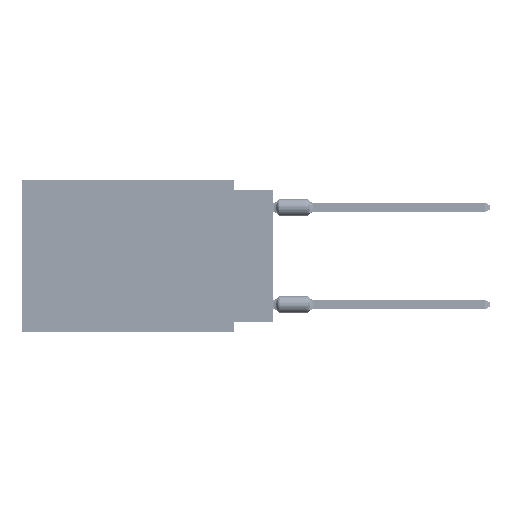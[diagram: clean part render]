
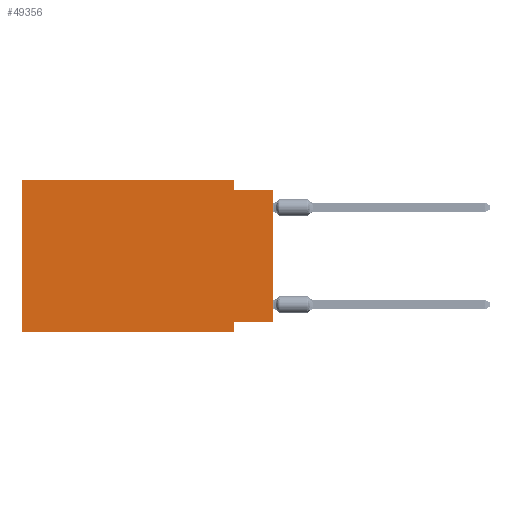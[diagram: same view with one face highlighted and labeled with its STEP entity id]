
A CAD part, left-side view. The second image highlights one B-rep face of the part: STEP entity #49356.
In plain terms, the highlighted planar face has unit normal (-1, 0, 0).
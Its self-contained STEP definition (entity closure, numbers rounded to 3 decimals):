
#107 = AXIS2_PLACEMENT_3D ( 'NONE', #959, #47826, #34821 ) ;
#242 = LINE ( 'NONE', #26298, #67312 ) ;
#959 = CARTESIAN_POINT ( 'NONE',  ( 0., 16.383, 0. ) ) ;
#1504 = LINE ( 'NONE', #49226, #22311 ) ;
#1626 = DIRECTION ( 'NONE',  ( 0., 0., -1. ) ) ;
#4898 = EDGE_CURVE ( 'NONE', #56116, #19500, #31081, .T. ) ;
#6947 = EDGE_CURVE ( 'NONE', #12516, #8193, #77338, .T. ) ;
#7441 = VECTOR ( 'NONE', #54636, 1000. ) ;
#7620 = VERTEX_POINT ( 'NONE', #11672 ) ;
#8193 = VERTEX_POINT ( 'NONE', #47993 ) ;
#10065 = LINE ( 'NONE', #30489, #33742 ) ;
#11672 = CARTESIAN_POINT ( 'NONE',  ( 0., 16.383, -9.906 ) ) ;
#11821 = VECTOR ( 'NONE', #30651, 1000. ) ;
#12516 = VERTEX_POINT ( 'NONE', #23083 ) ;
#12734 = EDGE_LOOP ( 'NONE', ( #46473, #35733, #55915, #79250, #60089, #73096, #34286, #26647 ) ) ;
#13983 = FACE_OUTER_BOUND ( 'NONE', #12734, .T. ) ;
#14127 = CARTESIAN_POINT ( 'NONE',  ( 0., 2.54, 0. ) ) ;
#14664 = CARTESIAN_POINT ( 'NONE',  ( 0., 2.54, -9.906 ) ) ;
#15011 = VECTOR ( 'NONE', #1626, 1000. ) ;
#16249 = DIRECTION ( 'NONE',  ( 0., -1., 0. ) ) ;
#16401 = CARTESIAN_POINT ( 'NONE',  ( 0., 2.54, 0. ) ) ;
#17886 = CARTESIAN_POINT ( 'NONE',  ( 0., 16.383, 0. ) ) ;
#19500 = VERTEX_POINT ( 'NONE', #69903 ) ;
#22311 = VECTOR ( 'NONE', #16249, 1000. ) ;
#22546 = EDGE_CURVE ( 'NONE', #7620, #52447, #10065, .T. ) ;
#22982 = LINE ( 'NONE', #56824, #74865 ) ;
#23083 = CARTESIAN_POINT ( 'NONE',  ( 0., 0., -9.271 ) ) ;
#23402 = EDGE_CURVE ( 'NONE', #31485, #56116, #75884, .T. ) ;
#26298 = CARTESIAN_POINT ( 'NONE',  ( 0., 16.383, 0. ) ) ;
#26647 = ORIENTED_EDGE ( 'NONE', *, *, #6947, .F. ) ;
#26649 = EDGE_CURVE ( 'NONE', #52447, #31485, #242, .T. ) ;
#30389 = VERTEX_POINT ( 'NONE', #74461 ) ;
#30489 = CARTESIAN_POINT ( 'NONE',  ( 0., 16.383, 0. ) ) ;
#30651 = DIRECTION ( 'NONE',  ( 0., -1., 0. ) ) ;
#31081 = LINE ( 'NONE', #45366, #11821 ) ;
#31485 = VERTEX_POINT ( 'NONE', #14127 ) ;
#31742 = DIRECTION ( 'NONE',  ( 0., 1., 0. ) ) ;
#33742 = VECTOR ( 'NONE', #36158, 1000. ) ;
#34286 = ORIENTED_EDGE ( 'NONE', *, *, #41299, .F. ) ;
#34821 = DIRECTION ( 'NONE',  ( 0., 0., -1. ) ) ;
#35733 = ORIENTED_EDGE ( 'NONE', *, *, #4898, .F. ) ;
#36158 = DIRECTION ( 'NONE',  ( 0., 0., 1. ) ) ;
#40480 = PLANE ( 'NONE',  #107 ) ;
#41049 = DIRECTION ( 'NONE',  ( 0., -1., 0. ) ) ;
#41299 = EDGE_CURVE ( 'NONE', #8193, #30389, #74145, .T. ) ;
#45366 = CARTESIAN_POINT ( 'NONE',  ( 0., 0., -0.635 ) ) ;
#46473 = ORIENTED_EDGE ( 'NONE', *, *, #64041, .T. ) ;
#47826 = DIRECTION ( 'NONE',  ( 1., 0., 0. ) ) ;
#47993 = CARTESIAN_POINT ( 'NONE',  ( 0., 2.54, -9.271 ) ) ;
#49226 = CARTESIAN_POINT ( 'NONE',  ( 0., 16.383, -9.906 ) ) ;
#49356 = ADVANCED_FACE ( 'NONE', ( #13983 ), #40480, .F. ) ;
#49453 = DIRECTION ( 'NONE',  ( 0., 0., 1. ) ) ;
#49528 = EDGE_CURVE ( 'NONE', #7620, #30389, #1504, .T. ) ;
#50655 = VECTOR ( 'NONE', #31742, 1000. ) ;
#52447 = VERTEX_POINT ( 'NONE', #17886 ) ;
#54636 = DIRECTION ( 'NONE',  ( 0., 0., -1. ) ) ;
#55915 = ORIENTED_EDGE ( 'NONE', *, *, #23402, .F. ) ;
#56116 = VERTEX_POINT ( 'NONE', #79734 ) ;
#56824 = CARTESIAN_POINT ( 'NONE',  ( 0., 0., 0. ) ) ;
#60089 = ORIENTED_EDGE ( 'NONE', *, *, #22546, .F. ) ;
#64041 = EDGE_CURVE ( 'NONE', #12516, #19500, #22982, .T. ) ;
#67312 = VECTOR ( 'NONE', #41049, 1000. ) ;
#69903 = CARTESIAN_POINT ( 'NONE',  ( 0., 0., -0.635 ) ) ;
#70398 = CARTESIAN_POINT ( 'NONE',  ( 0., 0., -9.271 ) ) ;
#73096 = ORIENTED_EDGE ( 'NONE', *, *, #49528, .T. ) ;
#74145 = LINE ( 'NONE', #14664, #15011 ) ;
#74461 = CARTESIAN_POINT ( 'NONE',  ( 0., 2.54, -9.906 ) ) ;
#74865 = VECTOR ( 'NONE', #49453, 1000. ) ;
#75884 = LINE ( 'NONE', #16401, #7441 ) ;
#77338 = LINE ( 'NONE', #70398, #50655 ) ;
#79250 = ORIENTED_EDGE ( 'NONE', *, *, #26649, .F. ) ;
#79734 = CARTESIAN_POINT ( 'NONE',  ( 0., 2.54, -0.635 ) ) ;
